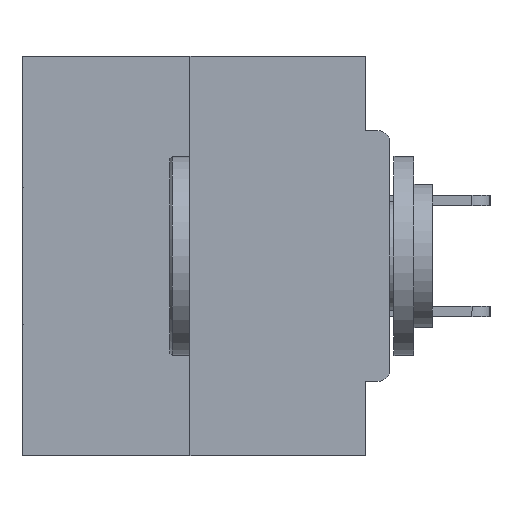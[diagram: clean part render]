
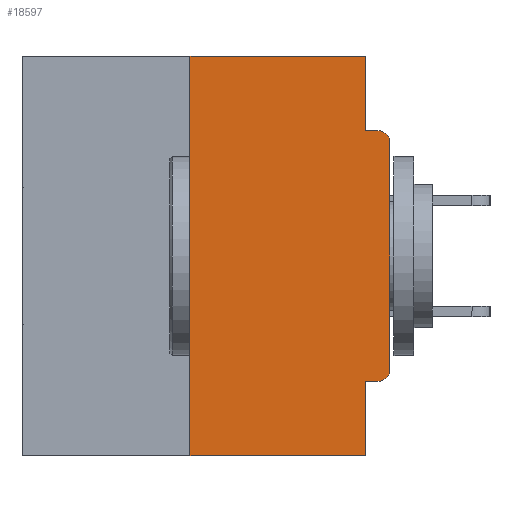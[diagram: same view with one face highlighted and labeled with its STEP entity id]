
A CAD part, left-side view. The second image highlights one B-rep face of the part: STEP entity #18597.
In plain terms, the highlighted planar face has unit normal (-1, 0, 0).
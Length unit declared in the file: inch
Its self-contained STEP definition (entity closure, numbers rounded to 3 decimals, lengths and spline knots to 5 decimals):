
#178 = VECTOR ( 'NONE', #9340, 39.37008 ) ;
#315 = VECTOR ( 'NONE', #12431, 39.37008 ) ;
#704 = VERTEX_POINT ( 'NONE', #17858 ) ;
#836 = CARTESIAN_POINT ( 'NONE',  ( 0., 0., -0.4065 ) ) ;
#1390 = DIRECTION ( 'NONE',  ( 0., 0., -1. ) ) ;
#1433 = CARTESIAN_POINT ( 'NONE',  ( 0., 0., 0. ) ) ;
#1976 = CARTESIAN_POINT ( 'NONE',  ( 0., 0.46, 0. ) ) ;
#2938 = CARTESIAN_POINT ( 'NONE',  ( 0., 0.46, -0.5 ) ) ;
#3045 = CARTESIAN_POINT ( 'NONE',  ( 0., 0.031, 0. ) ) ;
#3164 = LINE ( 'NONE', #10000, #11558 ) ;
#3697 = EDGE_CURVE ( 'NONE', #704, #21205, #33140, .T. ) ;
#4497 = EDGE_CURVE ( 'NONE', #9427, #18079, #33625, .T. ) ;
#4846 = LINE ( 'NONE', #36560, #178 ) ;
#5233 = DIRECTION ( 'NONE',  ( 1., 0., 0. ) ) ;
#5422 = CARTESIAN_POINT ( 'NONE',  ( 0., 0., -0.1085 ) ) ;
#6932 = VECTOR ( 'NONE', #19444, 39.37008 ) ;
#7427 = DIRECTION ( 'NONE',  ( 0., -1., 0. ) ) ;
#7815 = CARTESIAN_POINT ( 'NONE',  ( 0., 0., -0.0935 ) ) ;
#9340 = DIRECTION ( 'NONE',  ( 0., -1., 0. ) ) ;
#9427 = VERTEX_POINT ( 'NONE', #33174 ) ;
#10000 = CARTESIAN_POINT ( 'NONE',  ( 0., 0.031, 0. ) ) ;
#10147 = CARTESIAN_POINT ( 'NONE',  ( 0., 0.25, 0. ) ) ;
#10682 = VECTOR ( 'NONE', #36392, 39.37008 ) ;
#10713 = VERTEX_POINT ( 'NONE', #18389 ) ;
#11558 = VECTOR ( 'NONE', #1390, 39.37008 ) ;
#12431 = DIRECTION ( 'NONE',  ( 0., 1., 0. ) ) ;
#14259 = CARTESIAN_POINT ( 'NONE',  ( 0., 0., -0.3915 ) ) ;
#15354 = VERTEX_POINT ( 'NONE', #3045 ) ;
#16026 = DIRECTION ( 'NONE',  ( 0., 0., 1. ) ) ;
#16434 = EDGE_CURVE ( 'NONE', #15354, #10713, #3164, .T. ) ;
#16757 = CARTESIAN_POINT ( 'NONE',  ( 0., 0.015, -0.3915 ) ) ;
#16837 = EDGE_CURVE ( 'NONE', #25661, #35948, #33220, .T. ) ;
#16968 = PLANE ( 'NONE',  #31485 ) ;
#17473 = ORIENTED_EDGE ( 'NONE', *, *, #16434, .F. ) ;
#17586 = ORIENTED_EDGE ( 'NONE', *, *, #4497, .F. ) ;
#17682 = DIRECTION ( 'NONE',  ( 0., -1., 0. ) ) ;
#17858 = CARTESIAN_POINT ( 'NONE',  ( 0., 0.25, -0.5 ) ) ;
#18079 = VERTEX_POINT ( 'NONE', #20233 ) ;
#18194 = AXIS2_PLACEMENT_3D ( 'NONE', #16757, #25859, #28751 ) ;
#18209 = VERTEX_POINT ( 'NONE', #36268 ) ;
#18303 = VECTOR ( 'NONE', #17682, 39.37008 ) ;
#18389 = CARTESIAN_POINT ( 'NONE',  ( 0., 0.031, -0.0935 ) ) ;
#18399 = EDGE_CURVE ( 'NONE', #36555, #9427, #22767, .T. ) ;
#18597 = ADVANCED_FACE ( 'NONE', ( #19011 ), #16968, .F. ) ;
#18813 = CIRCLE ( 'NONE', #36927, 0.015 ) ;
#19011 = FACE_OUTER_BOUND ( 'NONE', #25915, .T. ) ;
#19444 = DIRECTION ( 'NONE',  ( 0., 0., 1. ) ) ;
#20000 = DIRECTION ( 'NONE',  ( -1., 0., 0. ) ) ;
#20233 = CARTESIAN_POINT ( 'NONE',  ( 0., 0.031, -0.5 ) ) ;
#20717 = EDGE_CURVE ( 'NONE', #21205, #15354, #4846, .T. ) ;
#20960 = EDGE_CURVE ( 'NONE', #36555, #25661, #36666, .T. ) ;
#21205 = VERTEX_POINT ( 'NONE', #37589 ) ;
#21545 = EDGE_CURVE ( 'NONE', #10713, #18209, #38471, .T. ) ;
#21756 = ORIENTED_EDGE ( 'NONE', *, *, #29426, .T. ) ;
#22304 = ORIENTED_EDGE ( 'NONE', *, *, #20717, .F. ) ;
#22767 = LINE ( 'NONE', #836, #315 ) ;
#22892 = DIRECTION ( 'NONE',  ( 0., 0., -1. ) ) ;
#22984 = DIRECTION ( 'NONE',  ( 0., 0., -1. ) ) ;
#23437 = ORIENTED_EDGE ( 'NONE', *, *, #16837, .T. ) ;
#23457 = CARTESIAN_POINT ( 'NONE',  ( 0., 0.015, -0.4065 ) ) ;
#23763 = ORIENTED_EDGE ( 'NONE', *, *, #30105, .T. ) ;
#23978 = LINE ( 'NONE', #2938, #18303 ) ;
#24460 = VECTOR ( 'NONE', #7427, 39.37008 ) ;
#25661 = VERTEX_POINT ( 'NONE', #14259 ) ;
#25859 = DIRECTION ( 'NONE',  ( -1., 0., 0. ) ) ;
#25915 = EDGE_LOOP ( 'NONE', ( #22304, #26198, #23763, #17586, #26563, #29890, #23437, #21756, #35391, #17473 ) ) ;
#26198 = ORIENTED_EDGE ( 'NONE', *, *, #3697, .F. ) ;
#26563 = ORIENTED_EDGE ( 'NONE', *, *, #18399, .F. ) ;
#28751 = DIRECTION ( 'NONE',  ( 0., 0., -1. ) ) ;
#29004 = CARTESIAN_POINT ( 'NONE',  ( 0., 0.031, -0.5 ) ) ;
#29426 = EDGE_CURVE ( 'NONE', #35948, #18209, #18813, .T. ) ;
#29890 = ORIENTED_EDGE ( 'NONE', *, *, #20960, .T. ) ;
#30105 = EDGE_CURVE ( 'NONE', #704, #18079, #23978, .T. ) ;
#31358 = VECTOR ( 'NONE', #16026, 39.37008 ) ;
#31485 = AXIS2_PLACEMENT_3D ( 'NONE', #1976, #5233, #22892 ) ;
#33140 = LINE ( 'NONE', #10147, #6932 ) ;
#33174 = CARTESIAN_POINT ( 'NONE',  ( 0., 0.031, -0.4065 ) ) ;
#33220 = LINE ( 'NONE', #1433, #31358 ) ;
#33625 = LINE ( 'NONE', #29004, #10682 ) ;
#35391 = ORIENTED_EDGE ( 'NONE', *, *, #21545, .F. ) ;
#35948 = VERTEX_POINT ( 'NONE', #5422 ) ;
#36268 = CARTESIAN_POINT ( 'NONE',  ( 0., 0.015, -0.0935 ) ) ;
#36392 = DIRECTION ( 'NONE',  ( 0., 0., -1. ) ) ;
#36555 = VERTEX_POINT ( 'NONE', #23457 ) ;
#36560 = CARTESIAN_POINT ( 'NONE',  ( 0., 0.46, 0. ) ) ;
#36666 = CIRCLE ( 'NONE', #18194, 0.015 ) ;
#36927 = AXIS2_PLACEMENT_3D ( 'NONE', #37902, #20000, #22984 ) ;
#37589 = CARTESIAN_POINT ( 'NONE',  ( 0., 0.25, 0. ) ) ;
#37902 = CARTESIAN_POINT ( 'NONE',  ( 0., 0.015, -0.1085 ) ) ;
#38471 = LINE ( 'NONE', #7815, #24460 ) ;
